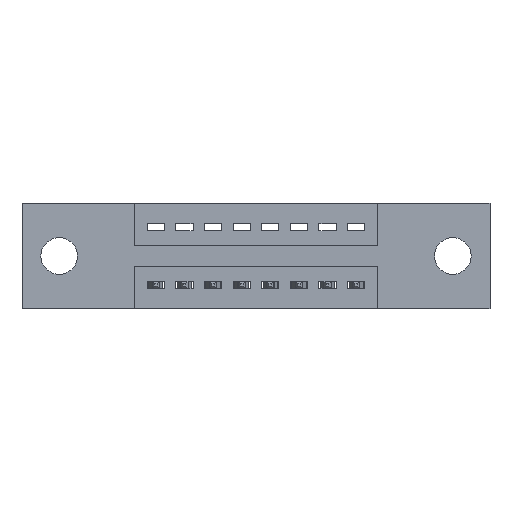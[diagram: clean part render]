
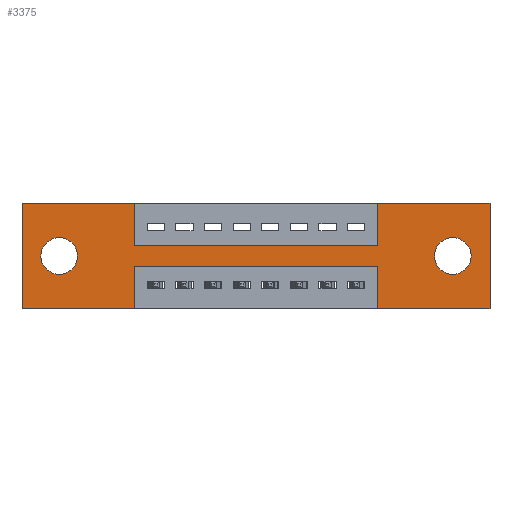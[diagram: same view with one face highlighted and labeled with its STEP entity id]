
A CAD part, front view. The second image highlights one B-rep face of the part: STEP entity #3375.
In plain terms, the highlighted planar face has unit normal (0, -1, 0).
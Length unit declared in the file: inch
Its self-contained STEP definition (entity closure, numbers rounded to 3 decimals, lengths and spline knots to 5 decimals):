
#98 = ORIENTED_EDGE ( 'NONE', *, *, #10576, .F. ) ;
#272 = DIRECTION ( 'NONE',  ( 0., 0., 1. ) ) ;
#276 = LINE ( 'NONE', #8608, #3875 ) ;
#290 = CARTESIAN_POINT ( 'NONE',  ( 1.635, 0., -0.37 ) ) ;
#377 = DIRECTION ( 'NONE',  ( 0., 1., 0. ) ) ;
#387 = CARTESIAN_POINT ( 'NONE',  ( 1.2425, 0., 0. ) ) ;
#541 = AXIS2_PLACEMENT_3D ( 'NONE', #6819, #2719, #8476 ) ;
#569 = AXIS2_PLACEMENT_3D ( 'NONE', #9698, #5772, #10508 ) ;
#581 = CIRCLE ( 'NONE', #569, 0.064 ) ;
#621 = ORIENTED_EDGE ( 'NONE', *, *, #7216, .F. ) ;
#787 = EDGE_CURVE ( 'NONE', #1886, #4844, #276, .T. ) ;
#874 = VECTOR ( 'NONE', #7715, 39.37008 ) ;
#941 = CARTESIAN_POINT ( 'NONE',  ( 0.3925, 0., 0. ) ) ;
#1064 = VERTEX_POINT ( 'NONE', #8220 ) ;
#1081 = VECTOR ( 'NONE', #272, 39.37008 ) ;
#1204 = ORIENTED_EDGE ( 'NONE', *, *, #6189, .F. ) ;
#1275 = VECTOR ( 'NONE', #4600, 39.37008 ) ;
#1411 = VECTOR ( 'NONE', #3002, 39.37008 ) ;
#1766 = ORIENTED_EDGE ( 'NONE', *, *, #4198, .T. ) ;
#1805 = VECTOR ( 'NONE', #9504, 39.37008 ) ;
#1886 = VERTEX_POINT ( 'NONE', #2835 ) ;
#1935 = EDGE_CURVE ( 'NONE', #5806, #10176, #5657, .T. ) ;
#1964 = DIRECTION ( 'NONE',  ( 0., 0., 1. ) ) ;
#1966 = AXIS2_PLACEMENT_3D ( 'NONE', #4586, #9410, #2849 ) ;
#2030 = DIRECTION ( 'NONE',  ( 1., 0., 0. ) ) ;
#2061 = LINE ( 'NONE', #5808, #4522 ) ;
#2130 = CARTESIAN_POINT ( 'NONE',  ( 1.635, 0., 0. ) ) ;
#2160 = VERTEX_POINT ( 'NONE', #5658 ) ;
#2164 = VERTEX_POINT ( 'NONE', #941 ) ;
#2260 = CARTESIAN_POINT ( 'NONE',  ( 1.2425, 0., 0. ) ) ;
#2263 = LINE ( 'NONE', #8781, #9582 ) ;
#2276 = CARTESIAN_POINT ( 'NONE',  ( 0., 0., 0. ) ) ;
#2278 = VERTEX_POINT ( 'NONE', #2638 ) ;
#2296 = LINE ( 'NONE', #8670, #1275 ) ;
#2503 = CARTESIAN_POINT ( 'NONE',  ( 0.13, 0., -0.121 ) ) ;
#2585 = CARTESIAN_POINT ( 'NONE',  ( 0., 0., 0. ) ) ;
#2638 = CARTESIAN_POINT ( 'NONE',  ( 1.505, 0., -0.249 ) ) ;
#2719 = DIRECTION ( 'NONE',  ( 0., 1., 0. ) ) ;
#2743 = CARTESIAN_POINT ( 'NONE',  ( 0.3925, 0., -0.22 ) ) ;
#2835 = CARTESIAN_POINT ( 'NONE',  ( 0.3925, 0., -0.22 ) ) ;
#2849 = DIRECTION ( 'NONE',  ( 0., 0., -1. ) ) ;
#2886 = EDGE_CURVE ( 'NONE', #10524, #1886, #5024, .T. ) ;
#2902 = VECTOR ( 'NONE', #4340, 39.37008 ) ;
#3002 = DIRECTION ( 'NONE',  ( 0., 0., 1. ) ) ;
#3131 = CARTESIAN_POINT ( 'NONE',  ( 0.3925, 0., -0.37 ) ) ;
#3169 = CARTESIAN_POINT ( 'NONE',  ( 1.2425, 0., -0.37 ) ) ;
#3203 = EDGE_CURVE ( 'NONE', #1064, #7067, #10475, .T. ) ;
#3274 = CIRCLE ( 'NONE', #6573, 0.064 ) ;
#3375 = ADVANCED_FACE ( 'NONE', ( #9063, #6785, #4741 ), #3765, .T. ) ;
#3441 = DIRECTION ( 'NONE',  ( 1., 0., 0. ) ) ;
#3685 = EDGE_LOOP ( 'NONE', ( #10262, #6369 ) ) ;
#3765 = PLANE ( 'NONE',  #1966 ) ;
#3875 = VECTOR ( 'NONE', #4678, 39.37008 ) ;
#3886 = VECTOR ( 'NONE', #9511, 39.37008 ) ;
#3957 = ORIENTED_EDGE ( 'NONE', *, *, #5145, .F. ) ;
#4198 = EDGE_CURVE ( 'NONE', #2278, #8912, #581, .T. ) ;
#4288 = ORIENTED_EDGE ( 'NONE', *, *, #10484, .T. ) ;
#4340 = DIRECTION ( 'NONE',  ( 0., 0., -1. ) ) ;
#4415 = LINE ( 'NONE', #387, #6313 ) ;
#4522 = VECTOR ( 'NONE', #3441, 39.37008 ) ;
#4586 = CARTESIAN_POINT ( 'NONE',  ( 0., 0., -0.37 ) ) ;
#4592 = ORIENTED_EDGE ( 'NONE', *, *, #4690, .F. ) ;
#4600 = DIRECTION ( 'NONE',  ( -1., 0., 0. ) ) ;
#4678 = DIRECTION ( 'NONE',  ( 0., 0., -1. ) ) ;
#4690 = EDGE_CURVE ( 'NONE', #2164, #6093, #5990, .T. ) ;
#4741 = FACE_OUTER_BOUND ( 'NONE', #5217, .T. ) ;
#4807 = EDGE_CURVE ( 'NONE', #7067, #1064, #3274, .T. ) ;
#4844 = VERTEX_POINT ( 'NONE', #3131 ) ;
#5024 = LINE ( 'NONE', #2743, #874 ) ;
#5145 = EDGE_CURVE ( 'NONE', #7683, #8023, #8897, .T. ) ;
#5217 = EDGE_LOOP ( 'NONE', ( #8470, #7484, #5763, #6170, #1204, #3957, #621, #5988, #4592, #98, #10410, #6014 ) ) ;
#5335 = CARTESIAN_POINT ( 'NONE',  ( 0.13, 0., -0.185 ) ) ;
#5630 = EDGE_CURVE ( 'NONE', #6135, #10524, #7366, .T. ) ;
#5657 = LINE ( 'NONE', #2276, #1411 ) ;
#5658 = CARTESIAN_POINT ( 'NONE',  ( 1.2425, 0., -0.15 ) ) ;
#5763 = ORIENTED_EDGE ( 'NONE', *, *, #5630, .F. ) ;
#5772 = DIRECTION ( 'NONE',  ( 0., 1., 0. ) ) ;
#5806 = VERTEX_POINT ( 'NONE', #6462 ) ;
#5808 = CARTESIAN_POINT ( 'NONE',  ( 0.3925, 0., -0.15 ) ) ;
#5838 = CARTESIAN_POINT ( 'NONE',  ( 0.3925, 0., -0.15 ) ) ;
#5988 = ORIENTED_EDGE ( 'NONE', *, *, #9011, .F. ) ;
#5990 = LINE ( 'NONE', #9232, #2902 ) ;
#6014 = ORIENTED_EDGE ( 'NONE', *, *, #9236, .F. ) ;
#6093 = VERTEX_POINT ( 'NONE', #5838 ) ;
#6135 = VERTEX_POINT ( 'NONE', #3169 ) ;
#6170 = ORIENTED_EDGE ( 'NONE', *, *, #9581, .F. ) ;
#6189 = EDGE_CURVE ( 'NONE', #8023, #6387, #6330, .T. ) ;
#6313 = VECTOR ( 'NONE', #7880, 39.37008 ) ;
#6330 = LINE ( 'NONE', #2130, #3886 ) ;
#6369 = ORIENTED_EDGE ( 'NONE', *, *, #3203, .T. ) ;
#6387 = VERTEX_POINT ( 'NONE', #290 ) ;
#6462 = CARTESIAN_POINT ( 'NONE',  ( 0., 0., -0.37 ) ) ;
#6478 = VECTOR ( 'NONE', #10049, 39.37008 ) ;
#6573 = AXIS2_PLACEMENT_3D ( 'NONE', #10232, #10258, #1964 ) ;
#6723 = CARTESIAN_POINT ( 'NONE',  ( 1.505, 0., -0.121 ) ) ;
#6785 = FACE_BOUND ( 'NONE', #3685, .T. ) ;
#6814 = CARTESIAN_POINT ( 'NONE',  ( 1.2425, 0., -0.37 ) ) ;
#6819 = CARTESIAN_POINT ( 'NONE',  ( 1.505, 0., -0.185 ) ) ;
#7067 = VERTEX_POINT ( 'NONE', #2503 ) ;
#7216 = EDGE_CURVE ( 'NONE', #2160, #7683, #4415, .T. ) ;
#7366 = LINE ( 'NONE', #6814, #1081 ) ;
#7484 = ORIENTED_EDGE ( 'NONE', *, *, #2886, .F. ) ;
#7683 = VERTEX_POINT ( 'NONE', #2260 ) ;
#7715 = DIRECTION ( 'NONE',  ( -1., 0., 0. ) ) ;
#7880 = DIRECTION ( 'NONE',  ( 0., 0., 1. ) ) ;
#8023 = VERTEX_POINT ( 'NONE', #10372 ) ;
#8220 = CARTESIAN_POINT ( 'NONE',  ( 0.13, 0., -0.249 ) ) ;
#8254 = CARTESIAN_POINT ( 'NONE',  ( 1.2425, 0., -0.22 ) ) ;
#8341 = CARTESIAN_POINT ( 'NONE',  ( 0., 0., 0. ) ) ;
#8470 = ORIENTED_EDGE ( 'NONE', *, *, #787, .F. ) ;
#8476 = DIRECTION ( 'NONE',  ( 0., 0., -1. ) ) ;
#8582 = EDGE_LOOP ( 'NONE', ( #4288, #1766 ) ) ;
#8608 = CARTESIAN_POINT ( 'NONE',  ( 0.3925, 0., -0.37 ) ) ;
#8640 = DIRECTION ( 'NONE',  ( 0., 0., 1. ) ) ;
#8647 = CARTESIAN_POINT ( 'NONE',  ( 0., 0., -0.37 ) ) ;
#8670 = CARTESIAN_POINT ( 'NONE',  ( 0., 0., -0.37 ) ) ;
#8781 = CARTESIAN_POINT ( 'NONE',  ( 0., 0., 0. ) ) ;
#8897 = LINE ( 'NONE', #2585, #6478 ) ;
#8912 = VERTEX_POINT ( 'NONE', #6723 ) ;
#9011 = EDGE_CURVE ( 'NONE', #6093, #2160, #2061, .T. ) ;
#9063 = FACE_BOUND ( 'NONE', #8582, .T. ) ;
#9087 = AXIS2_PLACEMENT_3D ( 'NONE', #5335, #377, #8640 ) ;
#9204 = CIRCLE ( 'NONE', #541, 0.064 ) ;
#9232 = CARTESIAN_POINT ( 'NONE',  ( 0.3925, 0., 0. ) ) ;
#9236 = EDGE_CURVE ( 'NONE', #4844, #5806, #10495, .T. ) ;
#9410 = DIRECTION ( 'NONE',  ( 0., -1., 0. ) ) ;
#9504 = DIRECTION ( 'NONE',  ( -1., 0., 0. ) ) ;
#9511 = DIRECTION ( 'NONE',  ( 0., 0., -1. ) ) ;
#9581 = EDGE_CURVE ( 'NONE', #6387, #6135, #2296, .T. ) ;
#9582 = VECTOR ( 'NONE', #2030, 39.37008 ) ;
#9698 = CARTESIAN_POINT ( 'NONE',  ( 1.505, 0., -0.185 ) ) ;
#10049 = DIRECTION ( 'NONE',  ( 1., 0., 0. ) ) ;
#10176 = VERTEX_POINT ( 'NONE', #8341 ) ;
#10232 = CARTESIAN_POINT ( 'NONE',  ( 0.13, 0., -0.185 ) ) ;
#10258 = DIRECTION ( 'NONE',  ( 0., 1., 0. ) ) ;
#10262 = ORIENTED_EDGE ( 'NONE', *, *, #4807, .T. ) ;
#10372 = CARTESIAN_POINT ( 'NONE',  ( 1.635, 0., 0. ) ) ;
#10410 = ORIENTED_EDGE ( 'NONE', *, *, #1935, .F. ) ;
#10475 = CIRCLE ( 'NONE', #9087, 0.064 ) ;
#10484 = EDGE_CURVE ( 'NONE', #8912, #2278, #9204, .T. ) ;
#10495 = LINE ( 'NONE', #8647, #1805 ) ;
#10508 = DIRECTION ( 'NONE',  ( 0., 0., -1. ) ) ;
#10524 = VERTEX_POINT ( 'NONE', #8254 ) ;
#10576 = EDGE_CURVE ( 'NONE', #10176, #2164, #2263, .T. ) ;
